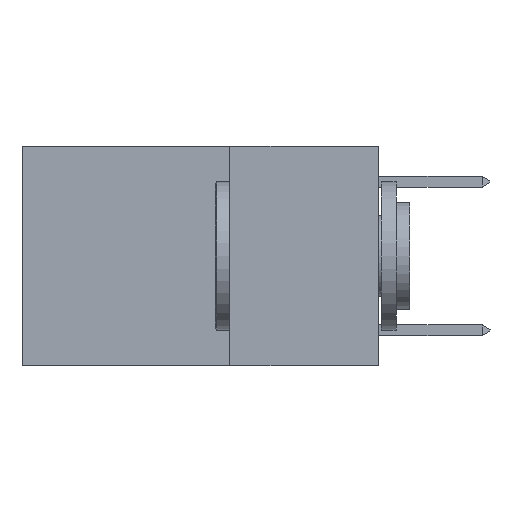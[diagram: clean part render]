
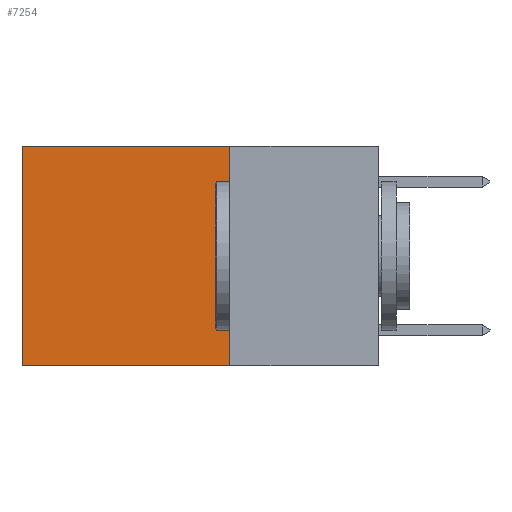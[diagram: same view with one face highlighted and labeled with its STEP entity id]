
A CAD part, left-side view. The second image highlights one B-rep face of the part: STEP entity #7254.
In plain terms, the highlighted planar face has unit normal (-1, 0, 0).
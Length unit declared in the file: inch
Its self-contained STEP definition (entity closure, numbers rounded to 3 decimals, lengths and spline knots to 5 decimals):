
#1162 = AXIS2_PLACEMENT_3D ( 'NONE', #17590, #5032, #11961 ) ;
#3768 = DIRECTION ( 'NONE',  ( 0., 1., 0. ) ) ;
#3770 = VECTOR ( 'NONE', #14707, 39.37008 ) ;
#3849 = EDGE_CURVE ( 'NONE', #17089, #5125, #12175, .T. ) ;
#4335 = ORIENTED_EDGE ( 'NONE', *, *, #13979, .F. ) ;
#4720 = CARTESIAN_POINT ( 'NONE',  ( 0.2625, 0.6, 0. ) ) ;
#5001 = CARTESIAN_POINT ( 'NONE',  ( 0.2625, 0.25, 0. ) ) ;
#5032 = DIRECTION ( 'NONE',  ( 1., 0., 0. ) ) ;
#5101 = VERTEX_POINT ( 'NONE', #8336 ) ;
#5125 = VERTEX_POINT ( 'NONE', #4720 ) ;
#5171 = EDGE_LOOP ( 'NONE', ( #11479, #4335, #14410, #12174 ) ) ;
#5484 = CARTESIAN_POINT ( 'NONE',  ( 0.2625, 0.25, -0.37 ) ) ;
#6038 = LINE ( 'NONE', #14272, #7414 ) ;
#6610 = EDGE_CURVE ( 'NONE', #17089, #8834, #15990, .T. ) ;
#6658 = LINE ( 'NONE', #11165, #15693 ) ;
#7254 = ADVANCED_FACE ( 'NONE', ( #14651 ), #16216, .F. ) ;
#7414 = VECTOR ( 'NONE', #17288, 39.37008 ) ;
#7447 = VECTOR ( 'NONE', #3768, 39.37008 ) ;
#8336 = CARTESIAN_POINT ( 'NONE',  ( 0.2625, 0.6, -0.37 ) ) ;
#8834 = VERTEX_POINT ( 'NONE', #5484 ) ;
#11165 = CARTESIAN_POINT ( 'NONE',  ( 0.2625, 0.25, -0.37 ) ) ;
#11479 = ORIENTED_EDGE ( 'NONE', *, *, #13391, .T. ) ;
#11961 = DIRECTION ( 'NONE',  ( 0., 0., -1. ) ) ;
#12174 = ORIENTED_EDGE ( 'NONE', *, *, #3849, .T. ) ;
#12175 = LINE ( 'NONE', #16433, #7447 ) ;
#12469 = DIRECTION ( 'NONE',  ( 0., 1., 0. ) ) ;
#13391 = EDGE_CURVE ( 'NONE', #5125, #5101, #6038, .T. ) ;
#13979 = EDGE_CURVE ( 'NONE', #8834, #5101, #6658, .T. ) ;
#14272 = CARTESIAN_POINT ( 'NONE',  ( 0.2625, 0.6, 0. ) ) ;
#14410 = ORIENTED_EDGE ( 'NONE', *, *, #6610, .F. ) ;
#14651 = FACE_OUTER_BOUND ( 'NONE', #5171, .T. ) ;
#14707 = DIRECTION ( 'NONE',  ( 0., 0., -1. ) ) ;
#15645 = CARTESIAN_POINT ( 'NONE',  ( 0.2625, 0.25, 0. ) ) ;
#15693 = VECTOR ( 'NONE', #12469, 39.37008 ) ;
#15990 = LINE ( 'NONE', #5001, #3770 ) ;
#16216 = PLANE ( 'NONE',  #1162 ) ;
#16433 = CARTESIAN_POINT ( 'NONE',  ( 0.2625, 0.25, 0. ) ) ;
#17089 = VERTEX_POINT ( 'NONE', #15645 ) ;
#17288 = DIRECTION ( 'NONE',  ( 0., 0., -1. ) ) ;
#17590 = CARTESIAN_POINT ( 'NONE',  ( 0.2625, 0.25, 0. ) ) ;
